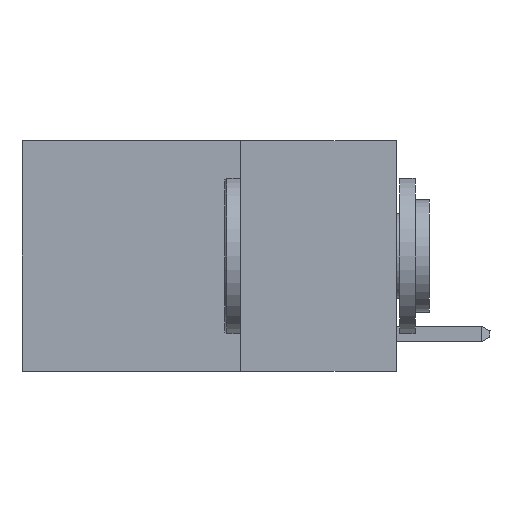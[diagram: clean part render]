
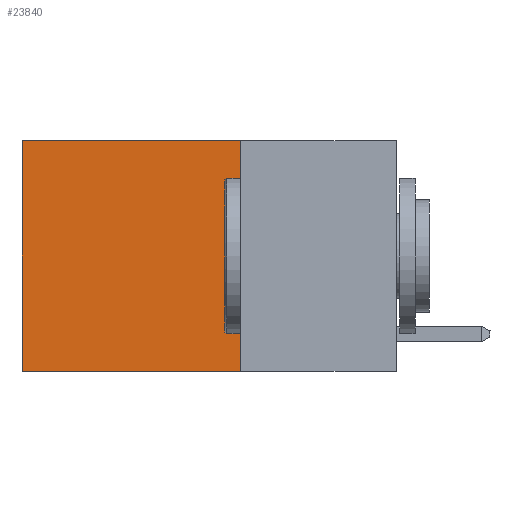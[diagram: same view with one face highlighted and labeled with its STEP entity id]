
A CAD part, left-side view. The second image highlights one B-rep face of the part: STEP entity #23840.
In plain terms, the highlighted planar face has unit normal (-1, 0, 0).
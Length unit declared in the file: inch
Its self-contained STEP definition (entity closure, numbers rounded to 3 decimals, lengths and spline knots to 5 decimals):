
#615 = CARTESIAN_POINT ( 'NONE',  ( 0.2625, 0.25, 0. ) ) ;
#645 = VERTEX_POINT ( 'NONE', #2576 ) ;
#2494 = EDGE_CURVE ( 'NONE', #22219, #15761, #10383, .T. ) ;
#2576 = CARTESIAN_POINT ( 'NONE',  ( 0.2625, 0.6, 0. ) ) ;
#4947 = ORIENTED_EDGE ( 'NONE', *, *, #5722, .F. ) ;
#5722 = EDGE_CURVE ( 'NONE', #15905, #22219, #11789, .T. ) ;
#6370 = VECTOR ( 'NONE', #18937, 39.37008 ) ;
#6955 = CARTESIAN_POINT ( 'NONE',  ( 0.2625, 0.25, 0. ) ) ;
#7403 = DIRECTION ( 'NONE',  ( 0., 0., -1. ) ) ;
#7970 = CARTESIAN_POINT ( 'NONE',  ( 0.2625, 0.25, 0. ) ) ;
#8094 = CARTESIAN_POINT ( 'NONE',  ( 0.2625, 0.6, -0.37 ) ) ;
#8574 = CARTESIAN_POINT ( 'NONE',  ( 0.2625, 0.25, -0.37 ) ) ;
#8865 = ORIENTED_EDGE ( 'NONE', *, *, #2494, .F. ) ;
#9626 = LINE ( 'NONE', #10712, #24160 ) ;
#10012 = DIRECTION ( 'NONE',  ( 0., 0., -1. ) ) ;
#10383 = LINE ( 'NONE', #12621, #20323 ) ;
#10712 = CARTESIAN_POINT ( 'NONE',  ( 0.2625, 0.25, 0. ) ) ;
#11789 = LINE ( 'NONE', #6955, #6370 ) ;
#12142 = FACE_OUTER_BOUND ( 'NONE', #24365, .T. ) ;
#12621 = CARTESIAN_POINT ( 'NONE',  ( 0.2625, 0.25, -0.37 ) ) ;
#13422 = EDGE_CURVE ( 'NONE', #15905, #645, #9626, .T. ) ;
#13676 = ORIENTED_EDGE ( 'NONE', *, *, #13422, .T. ) ;
#13873 = VECTOR ( 'NONE', #7403, 39.37008 ) ;
#14631 = DIRECTION ( 'NONE',  ( 0., 1., 0. ) ) ;
#14768 = ORIENTED_EDGE ( 'NONE', *, *, #16802, .T. ) ;
#15761 = VERTEX_POINT ( 'NONE', #8094 ) ;
#15905 = VERTEX_POINT ( 'NONE', #615 ) ;
#15947 = PLANE ( 'NONE',  #19200 ) ;
#16802 = EDGE_CURVE ( 'NONE', #645, #15761, #24321, .T. ) ;
#18937 = DIRECTION ( 'NONE',  ( 0., 0., -1. ) ) ;
#19200 = AXIS2_PLACEMENT_3D ( 'NONE', #7970, #21877, #10012 ) ;
#20323 = VECTOR ( 'NONE', #14631, 39.37008 ) ;
#21877 = DIRECTION ( 'NONE',  ( 1., 0., 0. ) ) ;
#22219 = VERTEX_POINT ( 'NONE', #8574 ) ;
#22549 = DIRECTION ( 'NONE',  ( 0., 1., 0. ) ) ;
#23227 = CARTESIAN_POINT ( 'NONE',  ( 0.2625, 0.6, 0. ) ) ;
#23840 = ADVANCED_FACE ( 'NONE', ( #12142 ), #15947, .F. ) ;
#24160 = VECTOR ( 'NONE', #22549, 39.37008 ) ;
#24321 = LINE ( 'NONE', #23227, #13873 ) ;
#24365 = EDGE_LOOP ( 'NONE', ( #14768, #8865, #4947, #13676 ) ) ;
